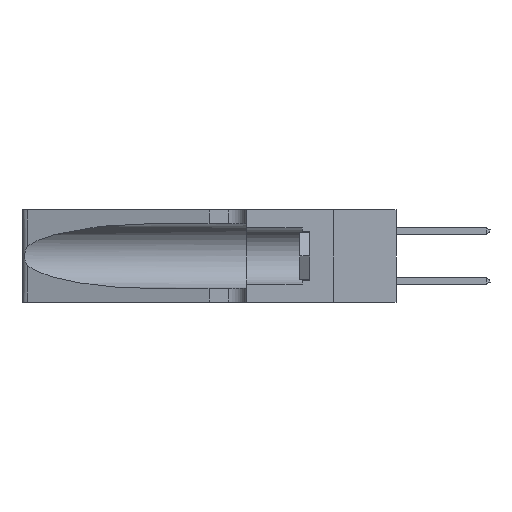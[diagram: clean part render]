
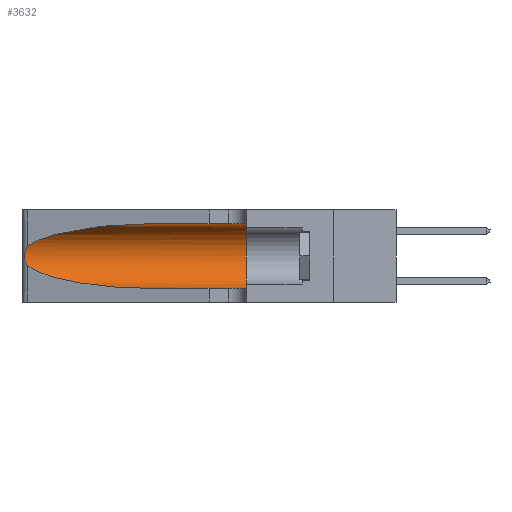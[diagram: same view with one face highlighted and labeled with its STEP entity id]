
A CAD part, left-side view. The second image highlights one B-rep face of the part: STEP entity #3632.
In plain terms, the highlighted cylindrical face has radius 3.308 mm (diameter 6.617 mm), a partial arc.
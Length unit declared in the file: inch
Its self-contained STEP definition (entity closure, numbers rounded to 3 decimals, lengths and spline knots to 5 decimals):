
#251 = DIRECTION ( 'NONE',  ( 0., -1., 0. ) ) ;
#857 =( BOUNDED_CURVE ( )  B_SPLINE_CURVE ( 3, ( #31976, #12182, #42022, #2303 ),
 .UNSPECIFIED., .F., .F. ) 
 B_SPLINE_CURVE_WITH_KNOTS ( ( 4, 4 ),
 ( 1.5708, 2.84003 ),
 .UNSPECIFIED. ) 
 CURVE ( )  GEOMETRIC_REPRESENTATION_ITEM ( )  RATIONAL_B_SPLINE_CURVE ( ( 1., 0.87, 0.87, 1. ) ) 
 REPRESENTATION_ITEM ( '' )  );
#2303 = CARTESIAN_POINT ( 'NONE',  ( 0.25487, 1.22718, 0.22369 ) ) ;
#3632 = ADVANCED_FACE ( 'NONE', ( #22191 ), #16509, .F. ) ;
#5686 = ORIENTED_EDGE ( 'NONE', *, *, #29733, .F. ) ;
#5793 = ORIENTED_EDGE ( 'NONE', *, *, #25959, .T. ) ;
#6405 = VECTOR ( 'NONE', #251, 39.37008 ) ;
#6508 = CARTESIAN_POINT ( 'NONE',  ( 0.1305, 1.61858, 0.05475 ) ) ;
#7620 = CARTESIAN_POINT ( 'NONE',  ( 0.25487, 1.22718, 0.22369 ) ) ;
#7702 = DIRECTION ( 'NONE',  ( 0., -1., 0. ) ) ;
#8680 = CARTESIAN_POINT ( 'NONE',  ( 0.1305, 0.35, 0.31525 ) ) ;
#9149 = CARTESIAN_POINT ( 'NONE',  ( 0.1305, 0.35, 0.185 ) ) ;
#10769 = CARTESIAN_POINT ( 'NONE',  ( 0.1305, 0.35, 0.05475 ) ) ;
#10890 = VECTOR ( 'NONE', #7702, 39.37008 ) ;
#11336 = VERTEX_POINT ( 'NONE', #10769 ) ;
#11496 = CARTESIAN_POINT ( 'NONE',  ( 0.1305, 0.72297, 0.31525 ) ) ;
#12182 = CARTESIAN_POINT ( 'NONE',  ( 0.18966, 0.96281, 0.31525 ) ) ;
#12775 = DIRECTION ( 'NONE',  ( 0., 0., 1. ) ) ;
#12984 = LINE ( 'NONE', #27696, #10890 ) ;
#15171 = CARTESIAN_POINT ( 'NONE',  ( 0.1305, 0.72297, 0.05475 ) ) ;
#15309 = CARTESIAN_POINT ( 'NONE',  ( 0.25555, 1.22993, 0.14849 ) ) ;
#15321 = CARTESIAN_POINT ( 'NONE',  ( 0.25487, 1.22718, 0.14631 ) ) ;
#15990 = DIRECTION ( 'NONE',  ( 0., 1., 0. ) ) ;
#16509 = CYLINDRICAL_SURFACE ( 'NONE', #42334, 0.13025 ) ;
#16552 = ORIENTED_EDGE ( 'NONE', *, *, #32601, .T. ) ;
#17670 = B_SPLINE_CURVE_WITH_KNOTS ( 'NONE', 3,
 ( #21786, #31906, #22233, #35512, #28459, #31600, #18614, #38583, #42245, #38424, #41957, #32051, #15309, #41668 ),
 .UNSPECIFIED., .F., .F.,
 ( 4, 2, 2, 2, 2, 2, 4 ),
 ( 0., 0.00027, 0.00053, 0.00107, 0.0016, 0.00187, 0.00214 ),
 .UNSPECIFIED. ) ;
#18340 = CARTESIAN_POINT ( 'NONE',  ( 0.18966, 0.96281, 0.05475 ) ) ;
#18614 = CARTESIAN_POINT ( 'NONE',  ( 0.26075, 1.23896, 0.19203 ) ) ;
#19287 = CARTESIAN_POINT ( 'NONE',  ( 0.1305, 1.61858, 0.185 ) ) ;
#19935 = EDGE_CURVE ( 'NONE', #39679, #11336, #34408, .T. ) ;
#21786 = CARTESIAN_POINT ( 'NONE',  ( 0.25487, 1.22718, 0.22369 ) ) ;
#22191 = FACE_OUTER_BOUND ( 'NONE', #35743, .T. ) ;
#22233 = CARTESIAN_POINT ( 'NONE',  ( 0.25639, 1.23184, 0.21858 ) ) ;
#23503 =( BOUNDED_CURVE ( )  B_SPLINE_CURVE ( 3, ( #15321, #41679, #18340, #15171 ),
 .UNSPECIFIED., .F., .F. ) 
 B_SPLINE_CURVE_WITH_KNOTS ( ( 4, 4 ),
 ( 3.44316, 4.71239 ),
 .UNSPECIFIED. ) 
 CURVE ( )  GEOMETRIC_REPRESENTATION_ITEM ( )  RATIONAL_B_SPLINE_CURVE ( ( 1., 0.87, 0.87, 1. ) ) 
 REPRESENTATION_ITEM ( '' )  );
#23707 = CARTESIAN_POINT ( 'NONE',  ( 0.25487, 1.22718, 0.14631 ) ) ;
#24540 = VERTEX_POINT ( 'NONE', #11496 ) ;
#25380 = VERTEX_POINT ( 'NONE', #8680 ) ;
#25959 = EDGE_CURVE ( 'NONE', #32317, #39679, #23503, .T. ) ;
#26763 = DIRECTION ( 'NONE',  ( 0., 0., -1. ) ) ;
#26835 = CIRCLE ( 'NONE', #32881, 0.13025 ) ;
#27047 = CARTESIAN_POINT ( 'NONE',  ( 0.1305, 0.72297, 0.05475 ) ) ;
#27696 = CARTESIAN_POINT ( 'NONE',  ( 0.1305, 1.61858, 0.31525 ) ) ;
#28459 = CARTESIAN_POINT ( 'NONE',  ( 0.25854, 1.2359, 0.20912 ) ) ;
#28876 = ORIENTED_EDGE ( 'NONE', *, *, #40529, .F. ) ;
#29733 = EDGE_CURVE ( 'NONE', #25380, #11336, #26835, .T. ) ;
#31600 = CARTESIAN_POINT ( 'NONE',  ( 0.26018, 1.23835, 0.19895 ) ) ;
#31906 = CARTESIAN_POINT ( 'NONE',  ( 0.25555, 1.22994, 0.2215 ) ) ;
#31976 = CARTESIAN_POINT ( 'NONE',  ( 0.1305, 0.72297, 0.31525 ) ) ;
#32051 = CARTESIAN_POINT ( 'NONE',  ( 0.25639, 1.23186, 0.15144 ) ) ;
#32317 = VERTEX_POINT ( 'NONE', #23707 ) ;
#32601 = EDGE_CURVE ( 'NONE', #24540, #38473, #857, .T. ) ;
#32701 = DIRECTION ( 'NONE',  ( 0., -1., 0. ) ) ;
#32881 = AXIS2_PLACEMENT_3D ( 'NONE', #9149, #15990, #12775 ) ;
#34408 = LINE ( 'NONE', #6508, #6405 ) ;
#35512 = CARTESIAN_POINT ( 'NONE',  ( 0.25787, 1.23484, 0.2124 ) ) ;
#35743 = EDGE_LOOP ( 'NONE', ( #16552, #38609, #5793, #36846, #5686, #28876 ) ) ;
#36846 = ORIENTED_EDGE ( 'NONE', *, *, #19935, .T. ) ;
#38424 = CARTESIAN_POINT ( 'NONE',  ( 0.25856, 1.23593, 0.16098 ) ) ;
#38473 = VERTEX_POINT ( 'NONE', #7620 ) ;
#38583 = CARTESIAN_POINT ( 'NONE',  ( 0.26075, 1.23896, 0.178 ) ) ;
#38609 = ORIENTED_EDGE ( 'NONE', *, *, #40669, .T. ) ;
#39679 = VERTEX_POINT ( 'NONE', #27047 ) ;
#40529 = EDGE_CURVE ( 'NONE', #24540, #25380, #12984, .T. ) ;
#40669 = EDGE_CURVE ( 'NONE', #38473, #32317, #17670, .T. ) ;
#41668 = CARTESIAN_POINT ( 'NONE',  ( 0.25487, 1.22718, 0.14631 ) ) ;
#41679 = CARTESIAN_POINT ( 'NONE',  ( 0.2373, 1.15595, 0.08982 ) ) ;
#41957 = CARTESIAN_POINT ( 'NONE',  ( 0.25789, 1.23486, 0.15765 ) ) ;
#42022 = CARTESIAN_POINT ( 'NONE',  ( 0.2373, 1.15595, 0.28018 ) ) ;
#42245 = CARTESIAN_POINT ( 'NONE',  ( 0.26017, 1.23833, 0.17102 ) ) ;
#42334 = AXIS2_PLACEMENT_3D ( 'NONE', #19287, #32701, #26763 ) ;
